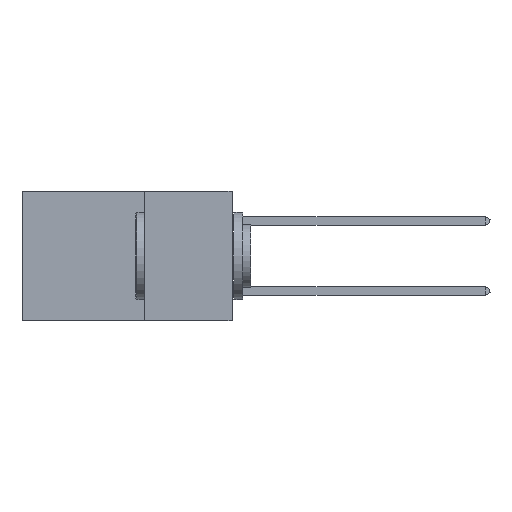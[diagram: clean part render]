
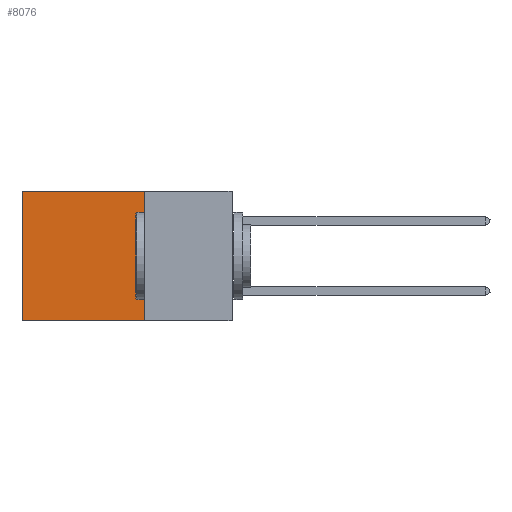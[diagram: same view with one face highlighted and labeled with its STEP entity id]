
A CAD part, left-side view. The second image highlights one B-rep face of the part: STEP entity #8076.
In plain terms, the highlighted planar face has unit normal (-1, 0, 0).
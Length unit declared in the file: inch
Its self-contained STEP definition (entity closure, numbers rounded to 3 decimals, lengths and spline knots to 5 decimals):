
#791 = ORIENTED_EDGE ( 'NONE', *, *, #17221, .T. ) ;
#2090 = CARTESIAN_POINT ( 'NONE',  ( 0.2875, 0.25, 0. ) ) ;
#3495 = CARTESIAN_POINT ( 'NONE',  ( 0.2875, 0.25, -0.37 ) ) ;
#3577 = CARTESIAN_POINT ( 'NONE',  ( 0.2875, 0.6, -0.37 ) ) ;
#3661 = CARTESIAN_POINT ( 'NONE',  ( 0.2875, 0.25, 0. ) ) ;
#3834 = CARTESIAN_POINT ( 'NONE',  ( 0.2875, 0.6, 0. ) ) ;
#4585 = LINE ( 'NONE', #2090, #23598 ) ;
#4627 = CARTESIAN_POINT ( 'NONE',  ( 0.2875, 0.25, -0.37 ) ) ;
#4786 = LINE ( 'NONE', #23519, #19546 ) ;
#5500 = DIRECTION ( 'NONE',  ( 1., 0., 0. ) ) ;
#6532 = EDGE_CURVE ( 'NONE', #21054, #20455, #11648, .T. ) ;
#6911 = CARTESIAN_POINT ( 'NONE',  ( 0.2875, 0.25, 0. ) ) ;
#7745 = ORIENTED_EDGE ( 'NONE', *, *, #21079, .F. ) ;
#8048 = FACE_OUTER_BOUND ( 'NONE', #20080, .T. ) ;
#8076 = ADVANCED_FACE ( 'NONE', ( #8048 ), #16627, .F. ) ;
#8331 = VERTEX_POINT ( 'NONE', #4627 ) ;
#8549 = VERTEX_POINT ( 'NONE', #3577 ) ;
#8847 = ORIENTED_EDGE ( 'NONE', *, *, #10410, .F. ) ;
#10410 = EDGE_CURVE ( 'NONE', #8331, #8549, #18170, .T. ) ;
#10741 = DIRECTION ( 'NONE',  ( 0., 0., -1. ) ) ;
#11648 = LINE ( 'NONE', #6911, #15933 ) ;
#15933 = VECTOR ( 'NONE', #21639, 39.37008 ) ;
#16474 = DIRECTION ( 'NONE',  ( 0., 1., 0. ) ) ;
#16627 = PLANE ( 'NONE',  #17833 ) ;
#17221 = EDGE_CURVE ( 'NONE', #20455, #8549, #4786, .T. ) ;
#17833 = AXIS2_PLACEMENT_3D ( 'NONE', #3661, #5500, #18470 ) ;
#18170 = LINE ( 'NONE', #3495, #18743 ) ;
#18470 = DIRECTION ( 'NONE',  ( 0., 0., -1. ) ) ;
#18528 = ORIENTED_EDGE ( 'NONE', *, *, #6532, .T. ) ;
#18743 = VECTOR ( 'NONE', #16474, 39.37008 ) ;
#18747 = DIRECTION ( 'NONE',  ( 0., 0., -1. ) ) ;
#19546 = VECTOR ( 'NONE', #10741, 39.37008 ) ;
#20080 = EDGE_LOOP ( 'NONE', ( #791, #8847, #7745, #18528 ) ) ;
#20455 = VERTEX_POINT ( 'NONE', #3834 ) ;
#20498 = CARTESIAN_POINT ( 'NONE',  ( 0.2875, 0.25, 0. ) ) ;
#21054 = VERTEX_POINT ( 'NONE', #20498 ) ;
#21079 = EDGE_CURVE ( 'NONE', #21054, #8331, #4585, .T. ) ;
#21639 = DIRECTION ( 'NONE',  ( 0., 1., 0. ) ) ;
#23519 = CARTESIAN_POINT ( 'NONE',  ( 0.2875, 0.6, 0. ) ) ;
#23598 = VECTOR ( 'NONE', #18747, 39.37008 ) ;
